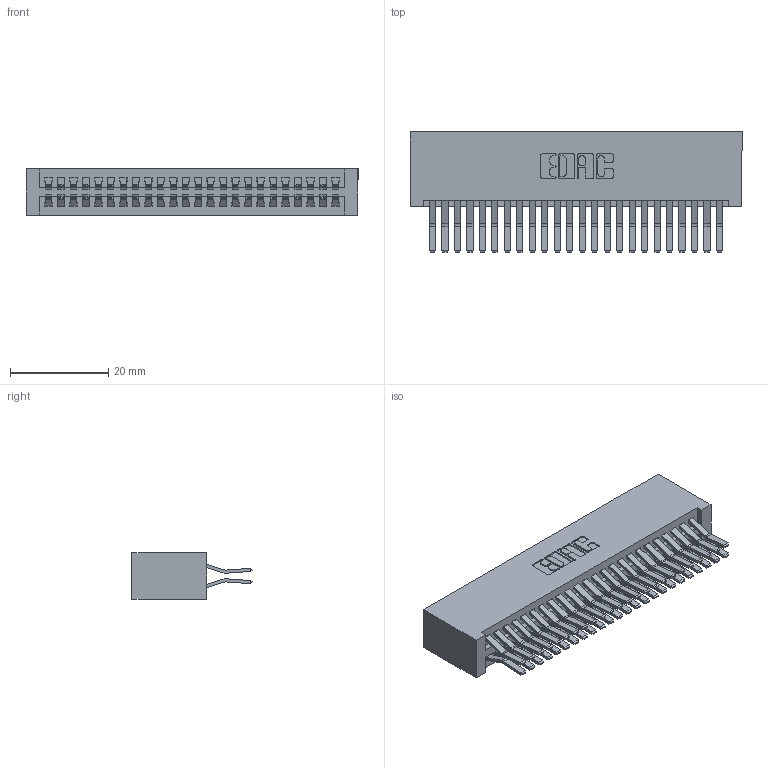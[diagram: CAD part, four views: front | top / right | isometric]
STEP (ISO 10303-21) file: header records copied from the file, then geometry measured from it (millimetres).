
FILE_DESCRIPTION (( 'STEP AP203' ), '1' );
FILE_NAME ('395-048-560-201.STEP', '2018-11-20T00:24:52', ( '' ), ( '' ), 'SwSTEP 2.0', 'SolidWorks 2016', '' );
FILE_SCHEMA (( 'CONFIG_CONTROL_DESIGN' ));
Length unit declared in the file: inch
Products named in the file (3): 345-292-001_560 Tail; 345 Part_No Mounting Lugs; 395-048-560-201
Assembly tree (49 placements, depth 2):
  395-048-560-201
    345 Part_No Mounting Lugs
    345-292-001_560 Tail  x48
Bounding box: 67.56 x 24.45 x 9.4 mm (x, y, z)
Volume: 7326.7 mm3; surface area: 11593.9 mm2
Topology: 49 solids, 49 shells, 2614 faces, 7757 edges, 5106 vertices
Faces by surface type: plane 1660, cylinder 954
Entity records: 21065 total; most frequent: CARTESIAN_POINT 3548, ORIENTED_EDGE 3482, DIRECTION 3149, EDGE_CURVE 1741, LINE 1517, VECTOR 1517, VERTEX_POINT 1158, AXIS2_PLACEMENT_3D 816
